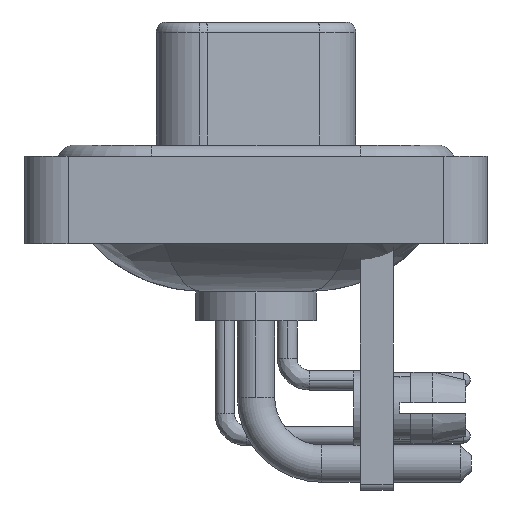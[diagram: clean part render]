
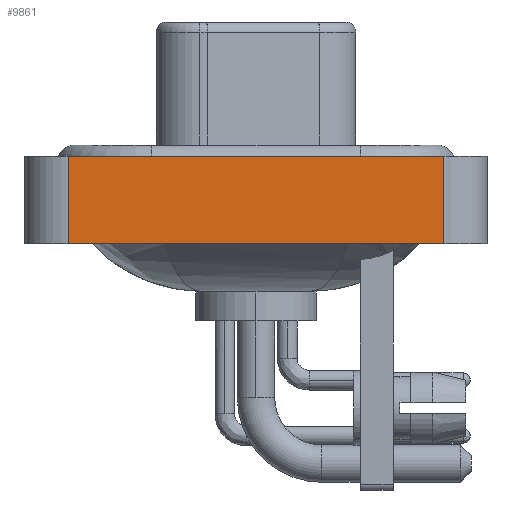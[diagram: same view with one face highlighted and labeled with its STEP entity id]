
A CAD part, left-side view. The second image highlights one B-rep face of the part: STEP entity #9861.
In plain terms, the highlighted planar face has unit normal (-1, 0, 0).
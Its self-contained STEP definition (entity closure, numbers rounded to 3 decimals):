
#1239 = CARTESIAN_POINT ( 'NONE',  ( -7.35, 8.55, -3.6 ) ) ;
#2032 = PLANE ( 'NONE',  #25771 ) ;
#3415 = CARTESIAN_POINT ( 'NONE',  ( -7.35, 8.55, -3.6 ) ) ;
#3590 = ORIENTED_EDGE ( 'NONE', *, *, #23541, .F. ) ;
#3703 = VERTEX_POINT ( 'NONE', #3415 ) ;
#3850 = VECTOR ( 'NONE', #26881, 1000. ) ;
#7869 = DIRECTION ( 'NONE',  ( 0., 0., 1. ) ) ;
#8026 = EDGE_CURVE ( 'NONE', #15715, #22153, #19944, .T. ) ;
#9204 = DIRECTION ( 'NONE',  ( 0., -1., 0. ) ) ;
#9292 = ORIENTED_EDGE ( 'NONE', *, *, #28486, .T. ) ;
#9393 = ORIENTED_EDGE ( 'NONE', *, *, #27985, .F. ) ;
#9861 = ADVANCED_FACE ( 'NONE', ( #22584 ), #2032, .T. ) ;
#10724 = VERTEX_POINT ( 'NONE', #19824 ) ;
#12993 = DIRECTION ( 'NONE',  ( -1., 0., 0. ) ) ;
#13275 = CARTESIAN_POINT ( 'NONE',  ( -7.35, -8.55, -3.6 ) ) ;
#14972 = VECTOR ( 'NONE', #7869, 1000. ) ;
#15557 = DIRECTION ( 'NONE',  ( 0., 0., 1. ) ) ;
#15715 = VERTEX_POINT ( 'NONE', #19411 ) ;
#16515 = VECTOR ( 'NONE', #19806, 1000. ) ;
#18177 = LINE ( 'NONE', #29124, #3850 ) ;
#19411 = CARTESIAN_POINT ( 'NONE',  ( -7.35, -8.55, -3.6 ) ) ;
#19806 = DIRECTION ( 'NONE',  ( 0., 0., 1. ) ) ;
#19824 = CARTESIAN_POINT ( 'NONE',  ( -7.35, 8.55, 0.4 ) ) ;
#19944 = LINE ( 'NONE', #24611, #16515 ) ;
#20108 = VECTOR ( 'NONE', #9204, 1000. ) ;
#21515 = LINE ( 'NONE', #1239, #14972 ) ;
#22153 = VERTEX_POINT ( 'NONE', #29602 ) ;
#22584 = FACE_OUTER_BOUND ( 'NONE', #25926, .T. ) ;
#22697 = LINE ( 'NONE', #29162, #20108 ) ;
#23541 = EDGE_CURVE ( 'NONE', #3703, #10724, #21515, .T. ) ;
#24142 = ORIENTED_EDGE ( 'NONE', *, *, #8026, .T. ) ;
#24611 = CARTESIAN_POINT ( 'NONE',  ( -7.35, -8.55, -3.6 ) ) ;
#25771 = AXIS2_PLACEMENT_3D ( 'NONE', #13275, #12993, #15557 ) ;
#25926 = EDGE_LOOP ( 'NONE', ( #24142, #9393, #3590, #9292 ) ) ;
#26881 = DIRECTION ( 'NONE',  ( 0., -1., 0. ) ) ;
#27985 = EDGE_CURVE ( 'NONE', #10724, #22153, #22697, .T. ) ;
#28486 = EDGE_CURVE ( 'NONE', #3703, #15715, #18177, .T. ) ;
#29124 = CARTESIAN_POINT ( 'NONE',  ( -7.35, -8.55, -3.6 ) ) ;
#29162 = CARTESIAN_POINT ( 'NONE',  ( -7.35, -8.55, 0.4 ) ) ;
#29602 = CARTESIAN_POINT ( 'NONE',  ( -7.35, -8.55, 0.4 ) ) ;
